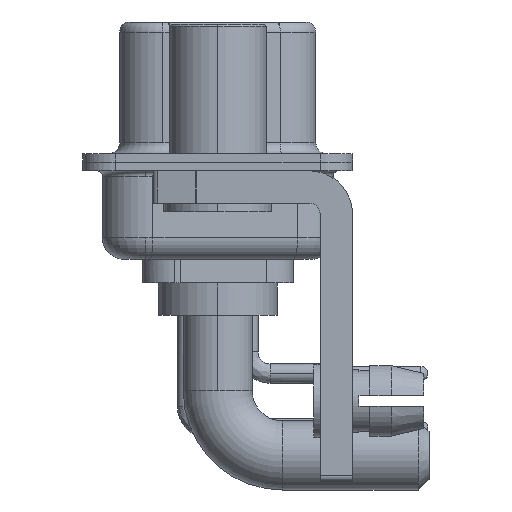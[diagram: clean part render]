
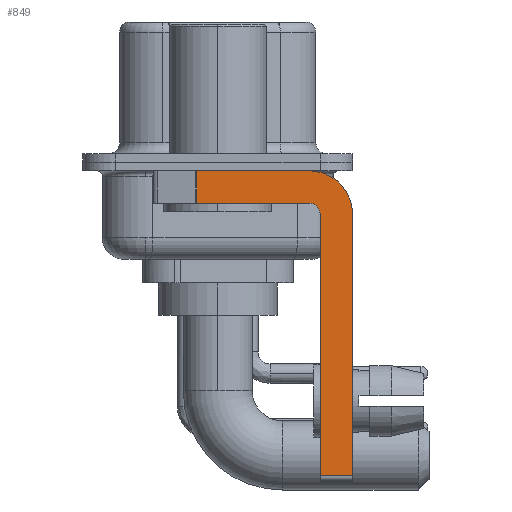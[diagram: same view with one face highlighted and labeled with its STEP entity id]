
A CAD part, left-side view. The second image highlights one B-rep face of the part: STEP entity #849.
In plain terms, the highlighted planar face has unit normal (-1, 0, 0).
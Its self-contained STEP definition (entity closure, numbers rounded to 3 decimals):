
#529 = LINE ( 'NONE', #19081, #7022 ) ;
#655 = EDGE_CURVE ( 'NONE', #13354, #24242, #19591, .T. ) ;
#711 = ORIENTED_EDGE ( 'NONE', *, *, #1917, .F. ) ;
#849 = ADVANCED_FACE ( 'NONE', ( #27687 ), #25444, .F. ) ;
#941 = VECTOR ( 'NONE', #21253, 1000. ) ;
#1788 = AXIS2_PLACEMENT_3D ( 'NONE', #7322, #14244, #16497 ) ;
#1917 = EDGE_CURVE ( 'NONE', #18909, #18212, #7728, .T. ) ;
#2311 = EDGE_CURVE ( 'NONE', #12519, #26341, #4826, .T. ) ;
#2428 = LINE ( 'NONE', #16607, #941 ) ;
#3700 = EDGE_LOOP ( 'NONE', ( #11498, #19668, #25050, #4482, #20129, #12295, #711, #7769 ) ) ;
#3735 = LINE ( 'NONE', #8002, #15270 ) ;
#3894 = VECTOR ( 'NONE', #14059, 1000. ) ;
#4014 = VECTOR ( 'NONE', #16167, 1000. ) ;
#4482 = ORIENTED_EDGE ( 'NONE', *, *, #655, .F. ) ;
#4826 = LINE ( 'NONE', #14314, #8222 ) ;
#4832 = CARTESIAN_POINT ( 'NONE',  ( -2.9, -4.25, -2.4 ) ) ;
#4860 = CARTESIAN_POINT ( 'NONE',  ( -2.9, -6.25, -2.4 ) ) ;
#6998 = CARTESIAN_POINT ( 'NONE',  ( -2.9, -4.75, -14.8 ) ) ;
#7022 = VECTOR ( 'NONE', #21327, 1000. ) ;
#7322 = CARTESIAN_POINT ( 'NONE',  ( -2.9, -4.25, -2.4 ) ) ;
#7564 = CARTESIAN_POINT ( 'NONE',  ( -2.9, -4.25, -2.4 ) ) ;
#7728 = LINE ( 'NONE', #4860, #3894 ) ;
#7769 = ORIENTED_EDGE ( 'NONE', *, *, #8348, .F. ) ;
#8002 = CARTESIAN_POINT ( 'NONE',  ( -2.9, 0.978, -1.9 ) ) ;
#8222 = VECTOR ( 'NONE', #28128, 1000. ) ;
#8348 = EDGE_CURVE ( 'NONE', #26341, #18909, #10617, .T. ) ;
#9464 = CARTESIAN_POINT ( 'NONE',  ( -2.9, -6.25, -2.4 ) ) ;
#9564 = EDGE_CURVE ( 'NONE', #25849, #18212, #2428, .T. ) ;
#10130 = DIRECTION ( 'NONE',  ( 1., 0., 0. ) ) ;
#10617 = CIRCLE ( 'NONE', #16323, 2. ) ;
#11011 = CARTESIAN_POINT ( 'NONE',  ( -2.9, -6.25, -14.55 ) ) ;
#11254 = CARTESIAN_POINT ( 'NONE',  ( -2.9, 0.978, -1.9 ) ) ;
#11429 = AXIS2_PLACEMENT_3D ( 'NONE', #4832, #16279, #22886 ) ;
#11498 = ORIENTED_EDGE ( 'NONE', *, *, #2311, .F. ) ;
#12295 = ORIENTED_EDGE ( 'NONE', *, *, #9564, .T. ) ;
#12519 = VERTEX_POINT ( 'NONE', #28018 ) ;
#13354 = VERTEX_POINT ( 'NONE', #25112 ) ;
#13457 = CARTESIAN_POINT ( 'NONE',  ( -2.9, -4.25, -0.4 ) ) ;
#13629 = LINE ( 'NONE', #6998, #4014 ) ;
#14059 = DIRECTION ( 'NONE',  ( 0., 0., -1. ) ) ;
#14244 = DIRECTION ( 'NONE',  ( -1., 0., 0. ) ) ;
#14314 = CARTESIAN_POINT ( 'NONE',  ( -2.9, 3., -0.4 ) ) ;
#14413 = EDGE_CURVE ( 'NONE', #25849, #13354, #13629, .T. ) ;
#15154 = VERTEX_POINT ( 'NONE', #11254 ) ;
#15270 = VECTOR ( 'NONE', #17162, 1000. ) ;
#15433 = CARTESIAN_POINT ( 'NONE',  ( -2.9, -4.75, -14.55 ) ) ;
#16167 = DIRECTION ( 'NONE',  ( 0., 0., 1. ) ) ;
#16279 = DIRECTION ( 'NONE',  ( 1., 0., 0. ) ) ;
#16323 = AXIS2_PLACEMENT_3D ( 'NONE', #7564, #10130, #26217 ) ;
#16497 = DIRECTION ( 'NONE',  ( 0., 0., 1. ) ) ;
#16607 = CARTESIAN_POINT ( 'NONE',  ( -2.9, -4.25, -14.55 ) ) ;
#17162 = DIRECTION ( 'NONE',  ( 0., 0., -1. ) ) ;
#18212 = VERTEX_POINT ( 'NONE', #11011 ) ;
#18909 = VERTEX_POINT ( 'NONE', #9464 ) ;
#18996 = EDGE_CURVE ( 'NONE', #24242, #15154, #529, .T. ) ;
#19081 = CARTESIAN_POINT ( 'NONE',  ( -2.9, -4.25, -1.9 ) ) ;
#19591 = CIRCLE ( 'NONE', #1788, 0.5 ) ;
#19668 = ORIENTED_EDGE ( 'NONE', *, *, #23211, .T. ) ;
#20129 = ORIENTED_EDGE ( 'NONE', *, *, #14413, .F. ) ;
#21253 = DIRECTION ( 'NONE',  ( 0., -1., 0. ) ) ;
#21327 = DIRECTION ( 'NONE',  ( 0., 1., 0. ) ) ;
#22886 = DIRECTION ( 'NONE',  ( 0., 0., -1. ) ) ;
#23211 = EDGE_CURVE ( 'NONE', #12519, #15154, #3735, .T. ) ;
#24242 = VERTEX_POINT ( 'NONE', #25151 ) ;
#25050 = ORIENTED_EDGE ( 'NONE', *, *, #18996, .F. ) ;
#25112 = CARTESIAN_POINT ( 'NONE',  ( -2.9, -4.75, -2.4 ) ) ;
#25151 = CARTESIAN_POINT ( 'NONE',  ( -2.9, -4.25, -1.9 ) ) ;
#25444 = PLANE ( 'NONE',  #11429 ) ;
#25849 = VERTEX_POINT ( 'NONE', #15433 ) ;
#26217 = DIRECTION ( 'NONE',  ( 0., 0., -1. ) ) ;
#26341 = VERTEX_POINT ( 'NONE', #13457 ) ;
#27687 = FACE_OUTER_BOUND ( 'NONE', #3700, .T. ) ;
#28018 = CARTESIAN_POINT ( 'NONE',  ( -2.9, 0.978, -0.4 ) ) ;
#28128 = DIRECTION ( 'NONE',  ( 0., -1., 0. ) ) ;
